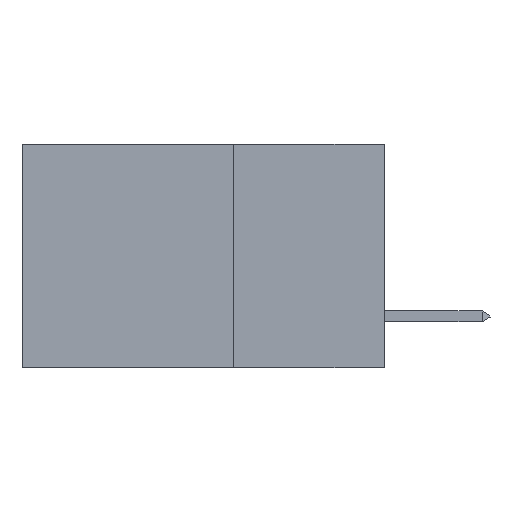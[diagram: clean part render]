
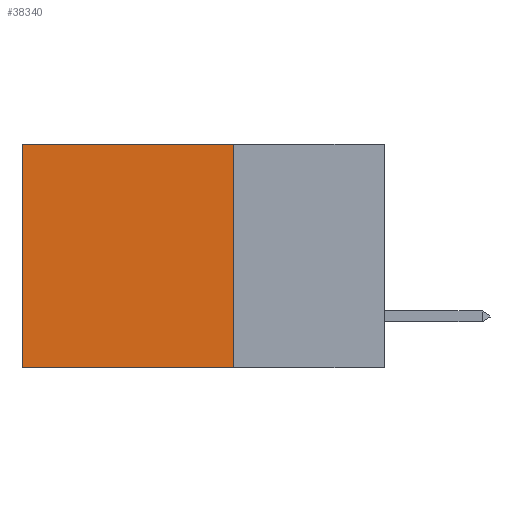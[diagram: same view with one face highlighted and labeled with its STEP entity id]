
A CAD part, left-side view. The second image highlights one B-rep face of the part: STEP entity #38340.
In plain terms, the highlighted planar face has unit normal (-1, 0, 0).
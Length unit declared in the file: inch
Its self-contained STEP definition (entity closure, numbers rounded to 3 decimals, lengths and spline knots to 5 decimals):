
#27 = VERTEX_POINT ( 'NONE', #39963 ) ;
#1582 = VECTOR ( 'NONE', #6437, 39.37008 ) ;
#2398 = EDGE_CURVE ( 'NONE', #26368, #41110, #2603, .T. ) ;
#2603 = LINE ( 'NONE', #29199, #31040 ) ;
#6437 = DIRECTION ( 'NONE',  ( 0., 0., -1. ) ) ;
#7545 = CARTESIAN_POINT ( 'NONE',  ( 0.2875, 0.25, 0. ) ) ;
#9230 = DIRECTION ( 'NONE',  ( 0., 1., 0. ) ) ;
#9976 = FACE_OUTER_BOUND ( 'NONE', #15894, .T. ) ;
#12760 = LINE ( 'NONE', #14197, #1582 ) ;
#14197 = CARTESIAN_POINT ( 'NONE',  ( 0.2875, 0.25, 0. ) ) ;
#15894 = EDGE_LOOP ( 'NONE', ( #45065, #18093, #26187, #34652 ) ) ;
#18093 = ORIENTED_EDGE ( 'NONE', *, *, #2398, .F. ) ;
#18456 = AXIS2_PLACEMENT_3D ( 'NONE', #7545, #28694, #39994 ) ;
#24921 = DIRECTION ( 'NONE',  ( 0., 1., 0. ) ) ;
#26187 = ORIENTED_EDGE ( 'NONE', *, *, #27183, .F. ) ;
#26368 = VERTEX_POINT ( 'NONE', #38871 ) ;
#26396 = DIRECTION ( 'NONE',  ( 0., 0., -1. ) ) ;
#26819 = CARTESIAN_POINT ( 'NONE',  ( 0.2875, 0.6, 0. ) ) ;
#27183 = EDGE_CURVE ( 'NONE', #27, #26368, #12760, .T. ) ;
#28585 = VECTOR ( 'NONE', #9230, 39.37008 ) ;
#28694 = DIRECTION ( 'NONE',  ( 1., 0., 0. ) ) ;
#29199 = CARTESIAN_POINT ( 'NONE',  ( 0.2875, 0.25, -0.37 ) ) ;
#31040 = VECTOR ( 'NONE', #24921, 39.37008 ) ;
#34652 = ORIENTED_EDGE ( 'NONE', *, *, #36877, .T. ) ;
#36877 = EDGE_CURVE ( 'NONE', #27, #39839, #41477, .T. ) ;
#38340 = ADVANCED_FACE ( 'NONE', ( #9976 ), #38781, .F. ) ;
#38601 = CARTESIAN_POINT ( 'NONE',  ( 0.2875, 0.6, -0.37 ) ) ;
#38781 = PLANE ( 'NONE',  #18456 ) ;
#38871 = CARTESIAN_POINT ( 'NONE',  ( 0.2875, 0.25, -0.37 ) ) ;
#39031 = VECTOR ( 'NONE', #26396, 39.37008 ) ;
#39839 = VERTEX_POINT ( 'NONE', #48008 ) ;
#39963 = CARTESIAN_POINT ( 'NONE',  ( 0.2875, 0.25, 0. ) ) ;
#39994 = DIRECTION ( 'NONE',  ( 0., 0., -1. ) ) ;
#41110 = VERTEX_POINT ( 'NONE', #38601 ) ;
#41193 = CARTESIAN_POINT ( 'NONE',  ( 0.2875, 0.25, 0. ) ) ;
#41477 = LINE ( 'NONE', #41193, #28585 ) ;
#41498 = EDGE_CURVE ( 'NONE', #39839, #41110, #50109, .T. ) ;
#45065 = ORIENTED_EDGE ( 'NONE', *, *, #41498, .T. ) ;
#48008 = CARTESIAN_POINT ( 'NONE',  ( 0.2875, 0.6, 0. ) ) ;
#50109 = LINE ( 'NONE', #26819, #39031 ) ;
